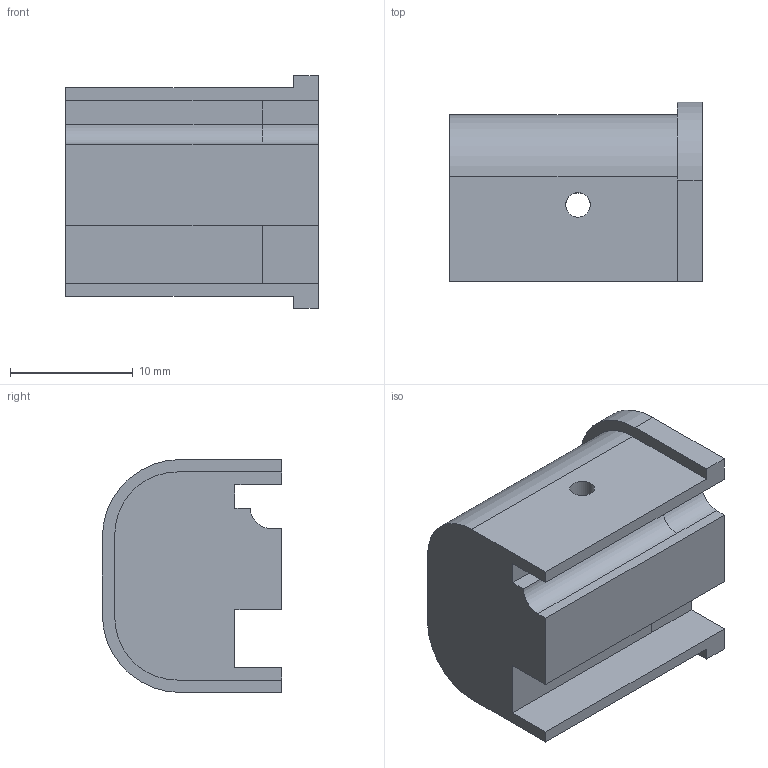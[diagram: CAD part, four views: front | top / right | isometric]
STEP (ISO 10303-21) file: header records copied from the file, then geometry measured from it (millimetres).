
FILE_DESCRIPTION(/* description */ (''),/* implementation_level */ '2;1');
FILE_NAME(/* name */ 'Halo Magnum Rear Plug.step',/* time_stamp */ '2022-03-30T10:09:34-06:00',/* author */ (''),/* organization */ (''),/* preprocessor_version */ 'ST-DEVELOPER v18.1',/* originating_system */ 'Autodesk Translation Framework v10.14.0.1471',/* authorisation */ '');
FILE_SCHEMA (('AUTOMOTIVE_DESIGN { 1 0 10303 214 3 1 1 }'));
Length unit declared in the file: millimetre
Products named in the file (1): Halo Magnum Beta
Bounding box: 20.57 x 14.61 x 18.96 mm (x, y, z)
Volume: 3931.9 mm3; surface area: 2047.6 mm2
Topology: 1 solids, 1 shells, 35 faces, 96 edges, 64 vertices
Faces by surface type: plane 26, cylinder 9
Full cylindrical faces by diameter (mm): 2 x1
Entity records: 1165 total; most frequent: CARTESIAN_POINT 196, ORIENTED_EDGE 192, DIRECTION 185, EDGE_CURVE 96, LINE 79, VECTOR 79, VERTEX_POINT 64, AXIS2_PLACEMENT_3D 53
